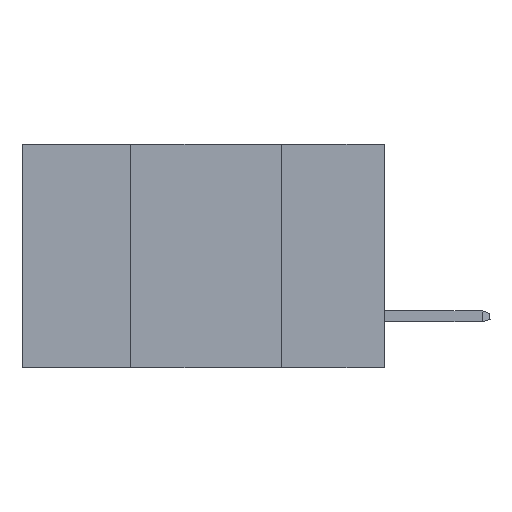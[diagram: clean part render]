
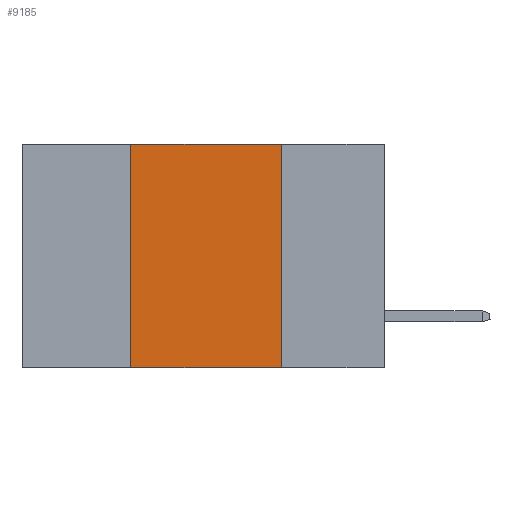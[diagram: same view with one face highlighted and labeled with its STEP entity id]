
A CAD part, left-side view. The second image highlights one B-rep face of the part: STEP entity #9185.
In plain terms, the highlighted planar face has unit normal (-1, 0, 0).
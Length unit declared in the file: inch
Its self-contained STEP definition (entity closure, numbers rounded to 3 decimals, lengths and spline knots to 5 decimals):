
#174 = DIRECTION ( 'NONE',  ( 1., 0., 0. ) ) ;
#588 = EDGE_LOOP ( 'NONE', ( #12319, #926, #16082, #17533 ) ) ;
#926 = ORIENTED_EDGE ( 'NONE', *, *, #14514, .F. ) ;
#1699 = DIRECTION ( 'NONE',  ( 0., 0., 1. ) ) ;
#3137 = CARTESIAN_POINT ( 'NONE',  ( 0., 0.42, -0.37 ) ) ;
#3154 = CARTESIAN_POINT ( 'NONE',  ( 0., 0.42, 0. ) ) ;
#3322 = CARTESIAN_POINT ( 'NONE',  ( 0., 0.6, 0. ) ) ;
#3930 = DIRECTION ( 'NONE',  ( 0., 0., -1. ) ) ;
#4453 = DIRECTION ( 'NONE',  ( 0., 0., -1. ) ) ;
#5046 = LINE ( 'NONE', #3322, #8515 ) ;
#5410 = EDGE_CURVE ( 'NONE', #7244, #9441, #13841, .T. ) ;
#6423 = DIRECTION ( 'NONE',  ( 0., -1., 0. ) ) ;
#6617 = CARTESIAN_POINT ( 'NONE',  ( 0., 0.6, -0.37 ) ) ;
#6902 = EDGE_CURVE ( 'NONE', #7244, #13681, #17313, .T. ) ;
#7244 = VERTEX_POINT ( 'NONE', #3137 ) ;
#8075 = DIRECTION ( 'NONE',  ( 0., -1., 0. ) ) ;
#8515 = VECTOR ( 'NONE', #6423, 39.37008 ) ;
#8707 = CARTESIAN_POINT ( 'NONE',  ( 0., 0.17, 0. ) ) ;
#9185 = ADVANCED_FACE ( 'NONE', ( #17931 ), #11695, .F. ) ;
#9198 = LINE ( 'NONE', #12840, #16909 ) ;
#9441 = VERTEX_POINT ( 'NONE', #11808 ) ;
#11319 = VECTOR ( 'NONE', #1699, 39.37008 ) ;
#11560 = AXIS2_PLACEMENT_3D ( 'NONE', #14650, #174, #4453 ) ;
#11614 = EDGE_CURVE ( 'NONE', #11674, #13681, #9198, .T. ) ;
#11674 = VERTEX_POINT ( 'NONE', #8707 ) ;
#11695 = PLANE ( 'NONE',  #11560 ) ;
#11808 = CARTESIAN_POINT ( 'NONE',  ( 0., 0.42, 0. ) ) ;
#12208 = VECTOR ( 'NONE', #8075, 39.37008 ) ;
#12319 = ORIENTED_EDGE ( 'NONE', *, *, #11614, .F. ) ;
#12840 = CARTESIAN_POINT ( 'NONE',  ( 0., 0.17, 0. ) ) ;
#13681 = VERTEX_POINT ( 'NONE', #19149 ) ;
#13841 = LINE ( 'NONE', #3154, #11319 ) ;
#14514 = EDGE_CURVE ( 'NONE', #9441, #11674, #5046, .T. ) ;
#14650 = CARTESIAN_POINT ( 'NONE',  ( 0., 0.6, 0. ) ) ;
#16082 = ORIENTED_EDGE ( 'NONE', *, *, #5410, .F. ) ;
#16909 = VECTOR ( 'NONE', #3930, 39.37008 ) ;
#17313 = LINE ( 'NONE', #6617, #12208 ) ;
#17533 = ORIENTED_EDGE ( 'NONE', *, *, #6902, .T. ) ;
#17931 = FACE_OUTER_BOUND ( 'NONE', #588, .T. ) ;
#19149 = CARTESIAN_POINT ( 'NONE',  ( 0., 0.17, -0.37 ) ) ;
